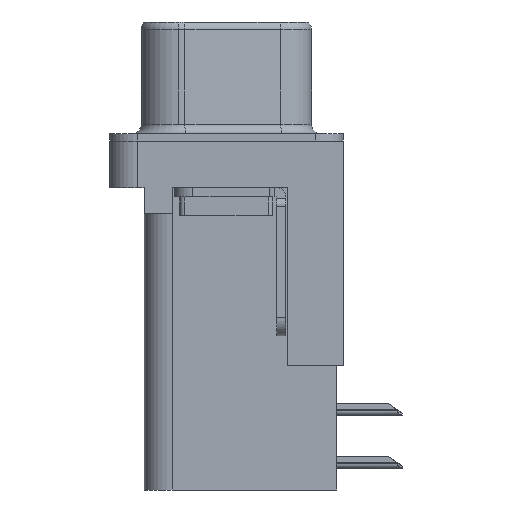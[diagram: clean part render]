
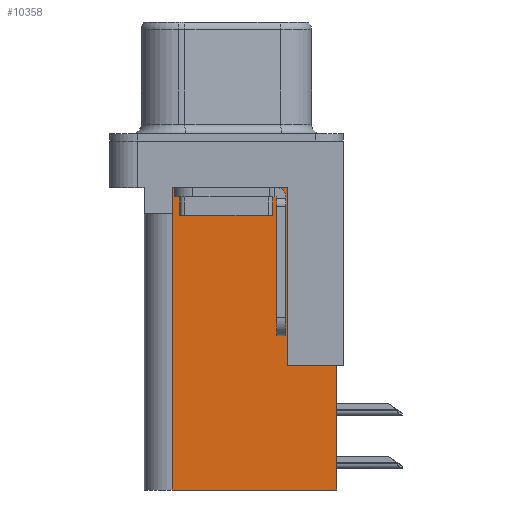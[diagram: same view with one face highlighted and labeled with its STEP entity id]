
A CAD part, left-side view. The second image highlights one B-rep face of the part: STEP entity #10358.
In plain terms, the highlighted planar face has unit normal (-1, 0, 0).
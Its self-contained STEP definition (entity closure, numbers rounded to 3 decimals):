
#78 = CARTESIAN_POINT ( 'NONE',  ( 3.7, -3.295, -18.76 ) ) ;
#244 = VERTEX_POINT ( 'NONE', #8078 ) ;
#514 = CARTESIAN_POINT ( 'NONE',  ( 3.7, -3.295, -18.76 ) ) ;
#595 = CARTESIAN_POINT ( 'NONE',  ( 3.7, 2.925, -18.76 ) ) ;
#829 = LINE ( 'NONE', #15920, #5218 ) ;
#1211 = VECTOR ( 'NONE', #3522, 1000. ) ;
#1594 = DIRECTION ( 'NONE',  ( 0., 0., 1. ) ) ;
#1624 = DIRECTION ( 'NONE',  ( 0., 1., 0. ) ) ;
#1810 = FACE_OUTER_BOUND ( 'NONE', #7889, .T. ) ;
#1875 = LINE ( 'NONE', #514, #13911 ) ;
#2535 = CARTESIAN_POINT ( 'NONE',  ( 3.7, -5.925, -12.05 ) ) ;
#3522 = DIRECTION ( 'NONE',  ( 0., 0., 1. ) ) ;
#3740 = ORIENTED_EDGE ( 'NONE', *, *, #20075, .T. ) ;
#4344 = CARTESIAN_POINT ( 'NONE',  ( 3.7, -3.295, -12.05 ) ) ;
#5218 = VECTOR ( 'NONE', #9648, 1000. ) ;
#5850 = ORIENTED_EDGE ( 'NONE', *, *, #11663, .T. ) ;
#7341 = EDGE_CURVE ( 'NONE', #13863, #12481, #1875, .T. ) ;
#7765 = PLANE ( 'NONE',  #14143 ) ;
#7889 = EDGE_LOOP ( 'NONE', ( #5850, #19764, #3740, #14507, #18522, #8332, #9105, #8838 ) ) ;
#8078 = CARTESIAN_POINT ( 'NONE',  ( 3.7, 2.895, -2.5 ) ) ;
#8332 = ORIENTED_EDGE ( 'NONE', *, *, #14142, .F. ) ;
#8444 = LINE ( 'NONE', #16964, #14821 ) ;
#8676 = DIRECTION ( 'NONE',  ( 0., 1., 0. ) ) ;
#8838 = ORIENTED_EDGE ( 'NONE', *, *, #17774, .T. ) ;
#9105 = ORIENTED_EDGE ( 'NONE', *, *, #16458, .T. ) ;
#9648 = DIRECTION ( 'NONE',  ( 0., 0., -1. ) ) ;
#9738 = DIRECTION ( 'NONE',  ( 0., 1., 0. ) ) ;
#10324 = VECTOR ( 'NONE', #1594, 1000. ) ;
#10358 = ADVANCED_FACE ( 'NONE', ( #1810 ), #7765, .F. ) ;
#10877 = VECTOR ( 'NONE', #8676, 1000. ) ;
#10968 = VERTEX_POINT ( 'NONE', #13366 ) ;
#10991 = CARTESIAN_POINT ( 'NONE',  ( 3.7, 2.925, -18.76 ) ) ;
#11254 = CARTESIAN_POINT ( 'NONE',  ( 3.7, 2.895, -3.9 ) ) ;
#11663 = EDGE_CURVE ( 'NONE', #16228, #244, #15511, .T. ) ;
#12192 = EDGE_CURVE ( 'NONE', #12481, #10968, #14030, .T. ) ;
#12469 = LINE ( 'NONE', #20354, #20259 ) ;
#12481 = VERTEX_POINT ( 'NONE', #595 ) ;
#12903 = CARTESIAN_POINT ( 'NONE',  ( 3.7, -3.295, -2.5 ) ) ;
#13299 = VERTEX_POINT ( 'NONE', #4344 ) ;
#13366 = CARTESIAN_POINT ( 'NONE',  ( 3.7, 2.925, -3.9 ) ) ;
#13809 = LINE ( 'NONE', #17400, #1211 ) ;
#13863 = VERTEX_POINT ( 'NONE', #18060 ) ;
#13877 = VERTEX_POINT ( 'NONE', #2535 ) ;
#13911 = VECTOR ( 'NONE', #19946, 1000. ) ;
#14030 = LINE ( 'NONE', #10991, #10324 ) ;
#14142 = EDGE_CURVE ( 'NONE', #13877, #13863, #829, .T. ) ;
#14143 = AXIS2_PLACEMENT_3D ( 'NONE', #78, #20231, #20212 ) ;
#14179 = VERTEX_POINT ( 'NONE', #11254 ) ;
#14472 = CARTESIAN_POINT ( 'NONE',  ( 3.7, -3.295, -2.5 ) ) ;
#14507 = ORIENTED_EDGE ( 'NONE', *, *, #12192, .F. ) ;
#14821 = VECTOR ( 'NONE', #18535, 1000. ) ;
#15057 = VECTOR ( 'NONE', #9738, 1000. ) ;
#15511 = LINE ( 'NONE', #14472, #15057 ) ;
#15920 = CARTESIAN_POINT ( 'NONE',  ( 3.7, -5.925, -2. ) ) ;
#16228 = VERTEX_POINT ( 'NONE', #12903 ) ;
#16458 = EDGE_CURVE ( 'NONE', #13877, #13299, #19200, .T. ) ;
#16964 = CARTESIAN_POINT ( 'NONE',  ( 3.7, 2.895, -3.9 ) ) ;
#17228 = EDGE_CURVE ( 'NONE', #244, #14179, #8444, .T. ) ;
#17400 = CARTESIAN_POINT ( 'NONE',  ( 3.7, -3.295, -18.76 ) ) ;
#17774 = EDGE_CURVE ( 'NONE', #13299, #16228, #13809, .T. ) ;
#18060 = CARTESIAN_POINT ( 'NONE',  ( 3.7, -5.925, -18.76 ) ) ;
#18522 = ORIENTED_EDGE ( 'NONE', *, *, #7341, .F. ) ;
#18535 = DIRECTION ( 'NONE',  ( 0., 0., -1. ) ) ;
#19200 = LINE ( 'NONE', #19522, #10877 ) ;
#19522 = CARTESIAN_POINT ( 'NONE',  ( 3.7, -6.295, -12.05 ) ) ;
#19764 = ORIENTED_EDGE ( 'NONE', *, *, #17228, .T. ) ;
#19946 = DIRECTION ( 'NONE',  ( 0., 1., 0. ) ) ;
#20075 = EDGE_CURVE ( 'NONE', #14179, #10968, #12469, .T. ) ;
#20212 = DIRECTION ( 'NONE',  ( 0., 1., 0. ) ) ;
#20231 = DIRECTION ( 'NONE',  ( 1., 0., 0. ) ) ;
#20259 = VECTOR ( 'NONE', #1624, 1000. ) ;
#20354 = CARTESIAN_POINT ( 'NONE',  ( 3.7, 0., -3.9 ) ) ;
